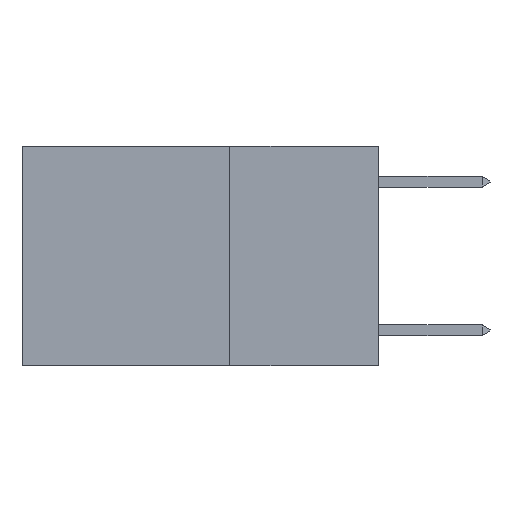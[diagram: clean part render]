
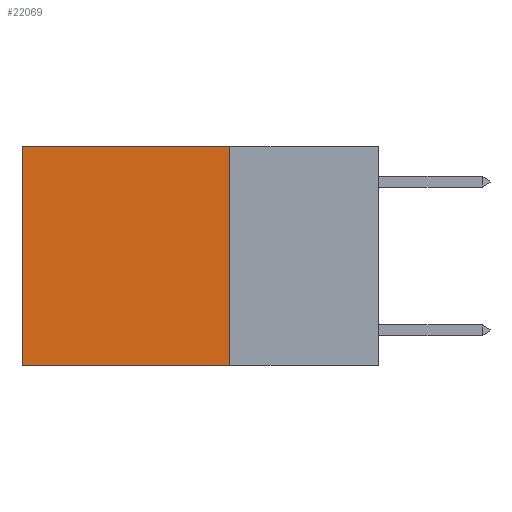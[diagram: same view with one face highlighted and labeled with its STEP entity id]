
A CAD part, left-side view. The second image highlights one B-rep face of the part: STEP entity #22069.
In plain terms, the highlighted planar face has unit normal (-1, 0, 0).
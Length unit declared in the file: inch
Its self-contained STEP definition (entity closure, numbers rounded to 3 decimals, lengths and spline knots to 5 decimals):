
#960 = CARTESIAN_POINT ( 'NONE',  ( 0.2625, 0.6, 0. ) ) ;
#1783 = VECTOR ( 'NONE', #16035, 39.37008 ) ;
#2382 = ORIENTED_EDGE ( 'NONE', *, *, #17856, .T. ) ;
#2824 = CARTESIAN_POINT ( 'NONE',  ( 0.2625, 0.25, -0.37 ) ) ;
#3971 = EDGE_CURVE ( 'NONE', #15845, #18220, #9318, .T. ) ;
#5205 = CARTESIAN_POINT ( 'NONE',  ( 0.2625, 0.25, 0. ) ) ;
#5495 = CARTESIAN_POINT ( 'NONE',  ( 0.2625, 0.25, 0. ) ) ;
#5951 = CARTESIAN_POINT ( 'NONE',  ( 0.2625, 0.25, 0. ) ) ;
#6065 = ORIENTED_EDGE ( 'NONE', *, *, #24467, .T. ) ;
#6325 = DIRECTION ( 'NONE',  ( 1., 0., 0. ) ) ;
#6378 = LINE ( 'NONE', #14248, #1783 ) ;
#6772 = EDGE_CURVE ( 'NONE', #18220, #12366, #19905, .T. ) ;
#6998 = VECTOR ( 'NONE', #8291, 39.37008 ) ;
#8291 = DIRECTION ( 'NONE',  ( 0., 1., 0. ) ) ;
#9318 = LINE ( 'NONE', #5205, #23673 ) ;
#11057 = VERTEX_POINT ( 'NONE', #960 ) ;
#12366 = VERTEX_POINT ( 'NONE', #15807 ) ;
#12395 = LINE ( 'NONE', #15893, #6998 ) ;
#14248 = CARTESIAN_POINT ( 'NONE',  ( 0.2625, 0.6, 0. ) ) ;
#15192 = ORIENTED_EDGE ( 'NONE', *, *, #6772, .F. ) ;
#15724 = CARTESIAN_POINT ( 'NONE',  ( 0.2625, 0.25, -0.37 ) ) ;
#15743 = PLANE ( 'NONE',  #20960 ) ;
#15807 = CARTESIAN_POINT ( 'NONE',  ( 0.2625, 0.6, -0.37 ) ) ;
#15845 = VERTEX_POINT ( 'NONE', #5495 ) ;
#15893 = CARTESIAN_POINT ( 'NONE',  ( 0.2625, 0.25, 0. ) ) ;
#16035 = DIRECTION ( 'NONE',  ( 0., 0., -1. ) ) ;
#17368 = ORIENTED_EDGE ( 'NONE', *, *, #3971, .F. ) ;
#17856 = EDGE_CURVE ( 'NONE', #15845, #11057, #12395, .T. ) ;
#18220 = VERTEX_POINT ( 'NONE', #2824 ) ;
#19905 = LINE ( 'NONE', #15724, #20480 ) ;
#19928 = FACE_OUTER_BOUND ( 'NONE', #23363, .T. ) ;
#20480 = VECTOR ( 'NONE', #23512, 39.37008 ) ;
#20736 = DIRECTION ( 'NONE',  ( 0., 0., -1. ) ) ;
#20960 = AXIS2_PLACEMENT_3D ( 'NONE', #5951, #6325, #21626 ) ;
#21626 = DIRECTION ( 'NONE',  ( 0., 0., -1. ) ) ;
#22069 = ADVANCED_FACE ( 'NONE', ( #19928 ), #15743, .F. ) ;
#23363 = EDGE_LOOP ( 'NONE', ( #6065, #15192, #17368, #2382 ) ) ;
#23512 = DIRECTION ( 'NONE',  ( 0., 1., 0. ) ) ;
#23673 = VECTOR ( 'NONE', #20736, 39.37008 ) ;
#24467 = EDGE_CURVE ( 'NONE', #11057, #12366, #6378, .T. ) ;
